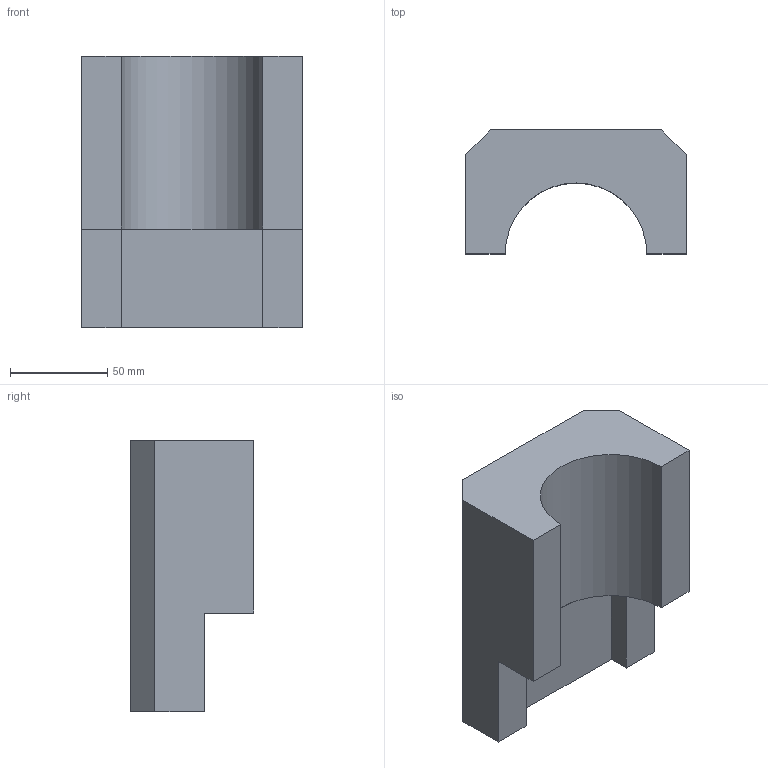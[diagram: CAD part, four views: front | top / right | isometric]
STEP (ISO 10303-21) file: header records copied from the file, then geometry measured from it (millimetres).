
FILE_DESCRIPTION (( 'STEP AP214' ), '1' );
FILE_NAME ('retainer.STEP', '2013-09-07T19:06:19', ( '' ), ( '' ), 'SwSTEP 2.0', 'SolidWorks 2013', '' );
FILE_SCHEMA (( 'AUTOMOTIVE_DESIGN' ));
Length unit declared in the file: inch
Products named in the file (1): retainer
Bounding box: 113.54 x 63.75 x 139.7 mm (x, y, z)
Volume: 605898.9 mm3; surface area: 63161.9 mm2
Topology: 1 solids, 1 shells, 25 faces, 68 edges, 45 vertices
Faces by surface type: plane 24, cylinder 1
Entity records: 817 total; most frequent: CARTESIAN_POINT 139, ORIENTED_EDGE 136, DIRECTION 123, EDGE_CURVE 68, VECTOR 65, LINE 65, VERTEX_POINT 45, AXIS2_PLACEMENT_3D 29
